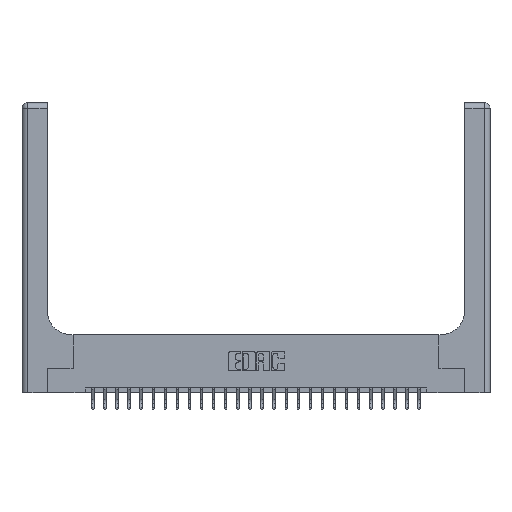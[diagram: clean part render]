
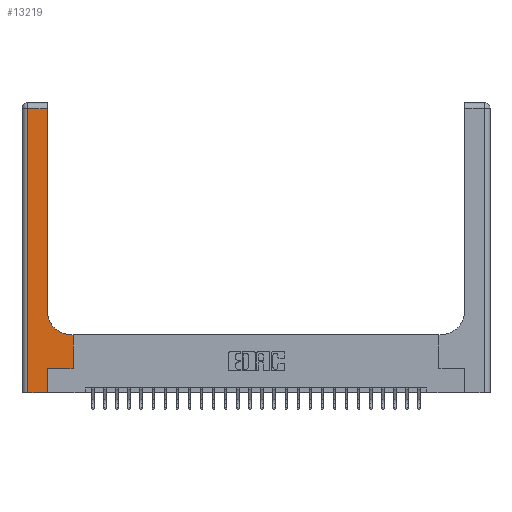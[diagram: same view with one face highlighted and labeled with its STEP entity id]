
A CAD part, top view. The second image highlights one B-rep face of the part: STEP entity #13219.
In plain terms, the highlighted planar face has unit normal (0, 0, 1).
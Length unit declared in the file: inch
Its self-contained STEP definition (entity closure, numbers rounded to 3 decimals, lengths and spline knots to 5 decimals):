
#257 = EDGE_CURVE ( 'NONE', #1041, #14631, #11107, .T. ) ;
#410 = VERTEX_POINT ( 'NONE', #20266 ) ;
#961 = LINE ( 'NONE', #21335, #10726 ) ;
#1041 = VERTEX_POINT ( 'NONE', #21852 ) ;
#1125 = CARTESIAN_POINT ( 'NONE',  ( 0.528, 0.25, 0.37 ) ) ;
#1299 = VECTOR ( 'NONE', #23144, 39.37008 ) ;
#1711 = CARTESIAN_POINT ( 'NONE',  ( 0., 3., 0.37 ) ) ;
#2124 = CARTESIAN_POINT ( 'NONE',  ( 0.06, 3., 0.37 ) ) ;
#3237 = DIRECTION ( 'NONE',  ( 1., 0., 0. ) ) ;
#3858 = VECTOR ( 'NONE', #19352, 39.37008 ) ;
#4100 = LINE ( 'NONE', #18104, #16501 ) ;
#4451 = VECTOR ( 'NONE', #5493, 39.37008 ) ;
#5096 = CARTESIAN_POINT ( 'NONE',  ( 0.06, 2.94, 0.37 ) ) ;
#5209 = ORIENTED_EDGE ( 'NONE', *, *, #22623, .T. ) ;
#5493 = DIRECTION ( 'NONE',  ( 0., 1., 0. ) ) ;
#5624 = CARTESIAN_POINT ( 'NONE',  ( 0.51, 0.85, 0.37 ) ) ;
#5943 = EDGE_CURVE ( 'NONE', #14631, #13089, #11073, .T. ) ;
#6065 = CARTESIAN_POINT ( 'NONE',  ( 0.528, 0.6, 0.37 ) ) ;
#6844 = VERTEX_POINT ( 'NONE', #7611 ) ;
#6995 = CARTESIAN_POINT ( 'NONE',  ( 0.265, 0., 0.37 ) ) ;
#7179 = DIRECTION ( 'NONE',  ( 0., 1., 0. ) ) ;
#7221 = CARTESIAN_POINT ( 'NONE',  ( 0.06, 0., 0.37 ) ) ;
#7405 = AXIS2_PLACEMENT_3D ( 'NONE', #5624, #17135, #3237 ) ;
#7611 = CARTESIAN_POINT ( 'NONE',  ( 0.26, 0.85, 0.37 ) ) ;
#7629 = EDGE_CURVE ( 'NONE', #6844, #410, #25052, .T. ) ;
#7918 = ORIENTED_EDGE ( 'NONE', *, *, #20805, .T. ) ;
#8497 = ORIENTED_EDGE ( 'NONE', *, *, #7629, .T. ) ;
#8611 = CARTESIAN_POINT ( 'NONE',  ( 0., 2.94, 0.37 ) ) ;
#8906 = VERTEX_POINT ( 'NONE', #7221 ) ;
#9247 = CARTESIAN_POINT ( 'NONE',  ( 0.26, 3., 0.37 ) ) ;
#9340 = EDGE_LOOP ( 'NONE', ( #8497, #5209, #17657, #7918, #24636, #16733, #25708, #16394, #19513 ) ) ;
#9447 = EDGE_CURVE ( 'NONE', #21503, #1041, #10360, .T. ) ;
#10313 = VECTOR ( 'NONE', #14233, 39.37008 ) ;
#10360 = LINE ( 'NONE', #10755, #14368 ) ;
#10726 = VECTOR ( 'NONE', #7179, 39.37008 ) ;
#10755 = CARTESIAN_POINT ( 'NONE',  ( 0.265, 0.25, 0.37 ) ) ;
#11073 = LINE ( 'NONE', #17091, #1299 ) ;
#11107 = LINE ( 'NONE', #1125, #4451 ) ;
#11453 = DIRECTION ( 'NONE',  ( -1., 0., 0. ) ) ;
#13089 = VERTEX_POINT ( 'NONE', #24738 ) ;
#13219 = ADVANCED_FACE ( 'NONE', ( #16535 ), #13435, .F. ) ;
#13435 = PLANE ( 'NONE',  #20357 ) ;
#14233 = DIRECTION ( 'NONE',  ( 0., -1., 0. ) ) ;
#14368 = VECTOR ( 'NONE', #22576, 39.37008 ) ;
#14399 = VERTEX_POINT ( 'NONE', #6995 ) ;
#14631 = VERTEX_POINT ( 'NONE', #6065 ) ;
#15744 = VECTOR ( 'NONE', #22663, 39.37008 ) ;
#16030 = EDGE_CURVE ( 'NONE', #24342, #8906, #21967, .T. ) ;
#16394 = ORIENTED_EDGE ( 'NONE', *, *, #5943, .T. ) ;
#16501 = VECTOR ( 'NONE', #24574, 39.37008 ) ;
#16535 = FACE_OUTER_BOUND ( 'NONE', #9340, .T. ) ;
#16733 = ORIENTED_EDGE ( 'NONE', *, *, #9447, .T. ) ;
#17091 = CARTESIAN_POINT ( 'NONE',  ( 0.26, 0.6, 0.37 ) ) ;
#17135 = DIRECTION ( 'NONE',  ( 0., 0., -1. ) ) ;
#17657 = ORIENTED_EDGE ( 'NONE', *, *, #16030, .T. ) ;
#18104 = CARTESIAN_POINT ( 'NONE',  ( 0., 0., 0.37 ) ) ;
#19099 = CIRCLE ( 'NONE', #7405, 0.25 ) ;
#19352 = DIRECTION ( 'NONE',  ( 0., 1., 0. ) ) ;
#19513 = ORIENTED_EDGE ( 'NONE', *, *, #22676, .T. ) ;
#19771 = CARTESIAN_POINT ( 'NONE',  ( 0.265, 0.25, 0.37 ) ) ;
#20266 = CARTESIAN_POINT ( 'NONE',  ( 0.26, 2.94, 0.37 ) ) ;
#20357 = AXIS2_PLACEMENT_3D ( 'NONE', #1711, #23395, #11453 ) ;
#20567 = LINE ( 'NONE', #8611, #15744 ) ;
#20805 = EDGE_CURVE ( 'NONE', #8906, #14399, #4100, .T. ) ;
#21335 = CARTESIAN_POINT ( 'NONE',  ( 0.265, 0., 0.37 ) ) ;
#21503 = VERTEX_POINT ( 'NONE', #19771 ) ;
#21852 = CARTESIAN_POINT ( 'NONE',  ( 0.528, 0.25, 0.37 ) ) ;
#21967 = LINE ( 'NONE', #2124, #10313 ) ;
#22576 = DIRECTION ( 'NONE',  ( 1., 0., 0. ) ) ;
#22623 = EDGE_CURVE ( 'NONE', #410, #24342, #20567, .T. ) ;
#22663 = DIRECTION ( 'NONE',  ( -1., 0., 0. ) ) ;
#22676 = EDGE_CURVE ( 'NONE', #13089, #6844, #19099, .T. ) ;
#22917 = EDGE_CURVE ( 'NONE', #14399, #21503, #961, .T. ) ;
#23144 = DIRECTION ( 'NONE',  ( -1., 0., 0. ) ) ;
#23395 = DIRECTION ( 'NONE',  ( 0., 0., -1. ) ) ;
#24342 = VERTEX_POINT ( 'NONE', #5096 ) ;
#24574 = DIRECTION ( 'NONE',  ( 1., 0., 0. ) ) ;
#24636 = ORIENTED_EDGE ( 'NONE', *, *, #22917, .T. ) ;
#24738 = CARTESIAN_POINT ( 'NONE',  ( 0.51, 0.6, 0.37 ) ) ;
#25052 = LINE ( 'NONE', #9247, #3858 ) ;
#25708 = ORIENTED_EDGE ( 'NONE', *, *, #257, .T. ) ;
